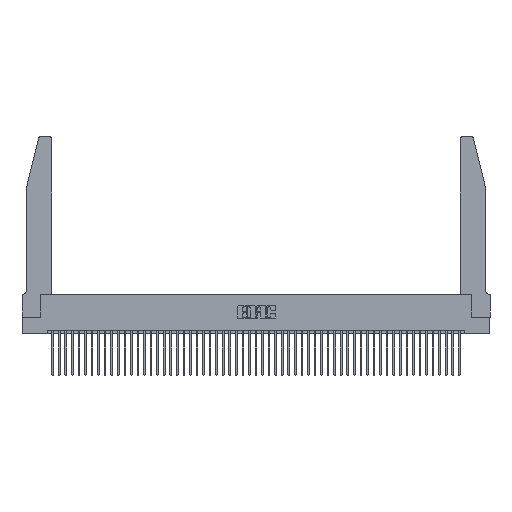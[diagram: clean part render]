
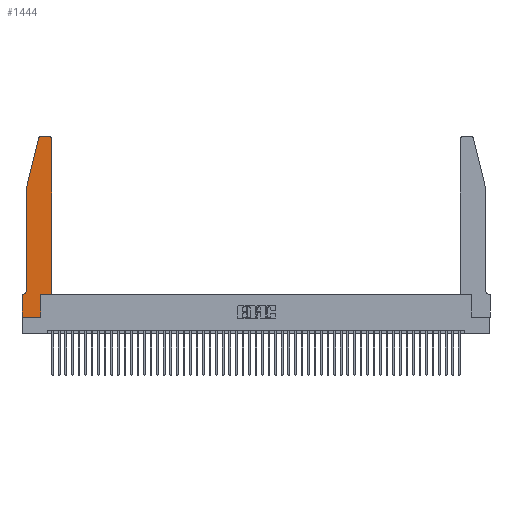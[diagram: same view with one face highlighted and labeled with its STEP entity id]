
A CAD part, top view. The second image highlights one B-rep face of the part: STEP entity #1444.
In plain terms, the highlighted planar face has unit normal (0, 0, 1).
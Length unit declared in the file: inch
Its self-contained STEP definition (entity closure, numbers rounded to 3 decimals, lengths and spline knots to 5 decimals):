
#878 = EDGE_CURVE ( 'NONE', #11981, #30749, #48204, .T. ) ;
#1444 = ADVANCED_FACE ( 'NONE', ( #27762 ), #15905, .T. ) ;
#2022 = EDGE_CURVE ( 'NONE', #49068, #17426, #47567, .T. ) ;
#2186 = VERTEX_POINT ( 'NONE', #9395 ) ;
#3033 = ORIENTED_EDGE ( 'NONE', *, *, #34875, .T. ) ;
#3345 = ORIENTED_EDGE ( 'NONE', *, *, #28360, .T. ) ;
#3566 = DIRECTION ( 'NONE',  ( 0., 0., 1. ) ) ;
#5417 = CARTESIAN_POINT ( 'NONE',  ( 0.4505, 0.35, 0.37 ) ) ;
#5724 = VERTEX_POINT ( 'NONE', #51161 ) ;
#5945 = EDGE_CURVE ( 'NONE', #39347, #24927, #25252, .T. ) ;
#5958 = CIRCLE ( 'NONE', #25693, 0.03 ) ;
#7221 = ORIENTED_EDGE ( 'NONE', *, *, #10913, .T. ) ;
#7633 = CARTESIAN_POINT ( 'NONE',  ( 0.0755, 0.42, 0.37 ) ) ;
#7718 = CARTESIAN_POINT ( 'NONE',  ( 0.2865, 0.35, 0.37 ) ) ;
#7848 = DIRECTION ( 'NONE',  ( -1., 0., 0. ) ) ;
#8030 = DIRECTION ( 'NONE',  ( 0., 0., -1. ) ) ;
#9395 = CARTESIAN_POINT ( 'NONE',  ( 0.25487, 2.72718, 0.37 ) ) ;
#9426 = ORIENTED_EDGE ( 'NONE', *, *, #46606, .T. ) ;
#9496 = VECTOR ( 'NONE', #26336, 39.37008 ) ;
#9975 = ORIENTED_EDGE ( 'NONE', *, *, #5945, .T. ) ;
#10847 = LINE ( 'NONE', #19196, #18948 ) ;
#10913 = EDGE_CURVE ( 'NONE', #5724, #39347, #26032, .T. ) ;
#10963 = CARTESIAN_POINT ( 'NONE',  ( 0.2605, 2.75, 0.37 ) ) ;
#11933 = AXIS2_PLACEMENT_3D ( 'NONE', #12984, #12798, #33113 ) ;
#11981 = VERTEX_POINT ( 'NONE', #36803 ) ;
#12798 = DIRECTION ( 'NONE',  ( 0., 0., 1. ) ) ;
#12810 = ORIENTED_EDGE ( 'NONE', *, *, #15436, .T. ) ;
#12984 = CARTESIAN_POINT ( 'NONE',  ( 0.4205, 2.72, 0.37 ) ) ;
#14148 = DIRECTION ( 'NONE',  ( 0., 0., 1. ) ) ;
#14698 = LINE ( 'NONE', #10963, #48853 ) ;
#14703 = LINE ( 'NONE', #7718, #32095 ) ;
#15436 = EDGE_CURVE ( 'NONE', #23014, #49068, #38691, .T. ) ;
#15578 = DIRECTION ( 'NONE',  ( 0., 1., 0. ) ) ;
#15905 = PLANE ( 'NONE',  #43403 ) ;
#16956 = EDGE_CURVE ( 'NONE', #2186, #23014, #36714, .T. ) ;
#17426 = VERTEX_POINT ( 'NONE', #34427 ) ;
#18287 = LINE ( 'NONE', #5417, #25093 ) ;
#18948 = VECTOR ( 'NONE', #39822, 39.37008 ) ;
#19196 = CARTESIAN_POINT ( 'NONE',  ( 0.0755, 0.35, 0.37 ) ) ;
#20021 = ORIENTED_EDGE ( 'NONE', *, *, #22776, .T. ) ;
#20624 = CARTESIAN_POINT ( 'NONE',  ( 0.4505, 2.72, 0.37 ) ) ;
#22266 = CARTESIAN_POINT ( 'NONE',  ( 0.284, 2.75, 0.37 ) ) ;
#22776 = EDGE_CURVE ( 'NONE', #30749, #36092, #37748, .T. ) ;
#23014 = VERTEX_POINT ( 'NONE', #37267 ) ;
#23903 = CARTESIAN_POINT ( 'NONE',  ( 0., 0., 0.37 ) ) ;
#24029 = DIRECTION ( 'NONE',  ( 1., 0., 0. ) ) ;
#24897 = VECTOR ( 'NONE', #43206, 39.37008 ) ;
#24927 = VERTEX_POINT ( 'NONE', #47548 ) ;
#25093 = VECTOR ( 'NONE', #44989, 39.37008 ) ;
#25252 = CIRCLE ( 'NONE', #11933, 0.03 ) ;
#25693 = AXIS2_PLACEMENT_3D ( 'NONE', #37922, #14148, #41891 ) ;
#26032 = LINE ( 'NONE', #42102, #29129 ) ;
#26336 = DIRECTION ( 'NONE',  ( 0., -1., 0. ) ) ;
#27321 = ORIENTED_EDGE ( 'NONE', *, *, #878, .T. ) ;
#27465 = DIRECTION ( 'NONE',  ( -1., 0., 0. ) ) ;
#27622 = CARTESIAN_POINT ( 'NONE',  ( 0., 0., 0.37 ) ) ;
#27662 = CARTESIAN_POINT ( 'NONE',  ( 0.0055, 0.42, 0.37 ) ) ;
#27762 = FACE_OUTER_BOUND ( 'NONE', #38251, .T. ) ;
#27888 = CARTESIAN_POINT ( 'NONE',  ( 0., 0.35, 0.37 ) ) ;
#28360 = EDGE_CURVE ( 'NONE', #36092, #31050, #14703, .T. ) ;
#29129 = VECTOR ( 'NONE', #34314, 39.37008 ) ;
#30749 = VERTEX_POINT ( 'NONE', #27622 ) ;
#31050 = VERTEX_POINT ( 'NONE', #31708 ) ;
#31391 = CARTESIAN_POINT ( 'NONE',  ( 0., 0., 0.37 ) ) ;
#31708 = CARTESIAN_POINT ( 'NONE',  ( 0.2865, 0.35, 0.37 ) ) ;
#32095 = VECTOR ( 'NONE', #15578, 39.37008 ) ;
#33113 = DIRECTION ( 'NONE',  ( 1., 0., 0. ) ) ;
#34314 = DIRECTION ( 'NONE',  ( 0., 1., 0. ) ) ;
#34427 = CARTESIAN_POINT ( 'NONE',  ( 0.0055, 0.35, 0.37 ) ) ;
#34875 = EDGE_CURVE ( 'NONE', #44224, #2186, #5958, .T. ) ;
#36092 = VERTEX_POINT ( 'NONE', #38293 ) ;
#36095 = ORIENTED_EDGE ( 'NONE', *, *, #2022, .T. ) ;
#36714 = LINE ( 'NONE', #46866, #24897 ) ;
#36803 = CARTESIAN_POINT ( 'NONE',  ( 0., 0.35, 0.37 ) ) ;
#37267 = CARTESIAN_POINT ( 'NONE',  ( 0.0755, 2., 0.37 ) ) ;
#37748 = LINE ( 'NONE', #23903, #45795 ) ;
#37922 = CARTESIAN_POINT ( 'NONE',  ( 0.284, 2.72, 0.37 ) ) ;
#38251 = EDGE_LOOP ( 'NONE', ( #43287, #3033, #44742, #12810, #36095, #50541, #27321, #20021, #3345, #9426, #7221, #9975 ) ) ;
#38293 = CARTESIAN_POINT ( 'NONE',  ( 0.2865, 0., 0.37 ) ) ;
#38462 = EDGE_CURVE ( 'NONE', #17426, #11981, #10847, .T. ) ;
#38691 = LINE ( 'NONE', #41966, #9496 ) ;
#39041 = DIRECTION ( 'NONE',  ( 0., -1., 0. ) ) ;
#39347 = VERTEX_POINT ( 'NONE', #20624 ) ;
#39822 = DIRECTION ( 'NONE',  ( -1., 0., 0. ) ) ;
#40727 = VECTOR ( 'NONE', #39041, 39.37008 ) ;
#40735 = AXIS2_PLACEMENT_3D ( 'NONE', #27662, #8030, #7848 ) ;
#41891 = DIRECTION ( 'NONE',  ( 1., 0., 0. ) ) ;
#41966 = CARTESIAN_POINT ( 'NONE',  ( 0.0755, 2., 0.37 ) ) ;
#42102 = CARTESIAN_POINT ( 'NONE',  ( 0.4505, 0.35, 0.37 ) ) ;
#43157 = EDGE_CURVE ( 'NONE', #24927, #44224, #14698, .T. ) ;
#43206 = DIRECTION ( 'NONE',  ( -0.239, -0.971, 0. ) ) ;
#43287 = ORIENTED_EDGE ( 'NONE', *, *, #43157, .T. ) ;
#43403 = AXIS2_PLACEMENT_3D ( 'NONE', #27888, #3566, #24029 ) ;
#44224 = VERTEX_POINT ( 'NONE', #22266 ) ;
#44742 = ORIENTED_EDGE ( 'NONE', *, *, #16956, .T. ) ;
#44989 = DIRECTION ( 'NONE',  ( 1., 0., 0. ) ) ;
#45795 = VECTOR ( 'NONE', #47370, 39.37008 ) ;
#46606 = EDGE_CURVE ( 'NONE', #31050, #5724, #18287, .T. ) ;
#46866 = CARTESIAN_POINT ( 'NONE',  ( 0.0755, 2., 0.37 ) ) ;
#47370 = DIRECTION ( 'NONE',  ( 1., 0., 0. ) ) ;
#47548 = CARTESIAN_POINT ( 'NONE',  ( 0.4205, 2.75, 0.37 ) ) ;
#47567 = CIRCLE ( 'NONE', #40735, 0.07 ) ;
#48204 = LINE ( 'NONE', #31391, #40727 ) ;
#48853 = VECTOR ( 'NONE', #27465, 39.37008 ) ;
#49068 = VERTEX_POINT ( 'NONE', #7633 ) ;
#50541 = ORIENTED_EDGE ( 'NONE', *, *, #38462, .T. ) ;
#51161 = CARTESIAN_POINT ( 'NONE',  ( 0.4505, 0.35, 0.37 ) ) ;
